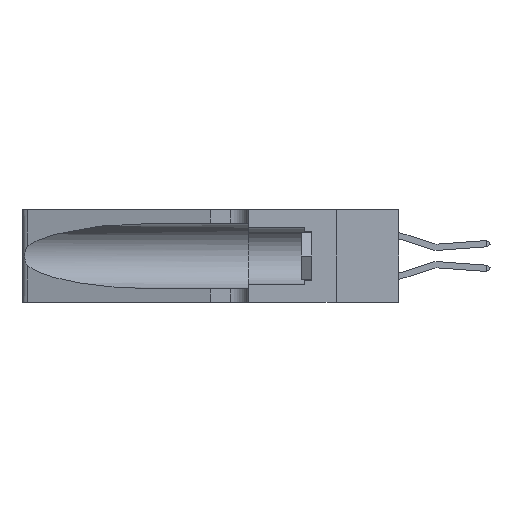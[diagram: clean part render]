
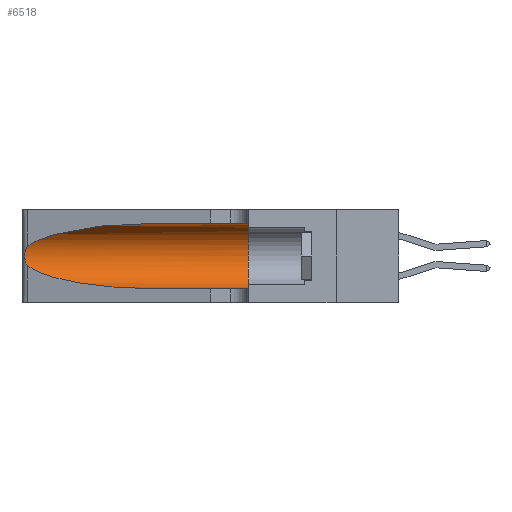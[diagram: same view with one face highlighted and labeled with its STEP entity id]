
A CAD part, left-side view. The second image highlights one B-rep face of the part: STEP entity #6518.
In plain terms, the highlighted cylindrical face has radius 3.308 mm (diameter 6.617 mm), a partial arc.
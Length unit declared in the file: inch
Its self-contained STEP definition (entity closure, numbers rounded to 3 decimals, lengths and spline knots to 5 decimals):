
#9 = B_SPLINE_CURVE_WITH_KNOTS ( 'NONE', 3,
 ( #10146, #8368, #3070, #15418, #4874, #17189, #6656, #18948, #8446, #20697, #10224, #22451, #12012, #1357 ),
 .UNSPECIFIED., .F., .F.,
 ( 4, 2, 2, 2, 2, 2, 4 ),
 ( 0., 0.00027, 0.00053, 0.00107, 0.0016, 0.00187, 0.00214 ),
 .UNSPECIFIED. ) ;
#262 = DIRECTION ( 'NONE',  ( 0., 1., 0. ) ) ;
#530 = AXIS2_PLACEMENT_3D ( 'NONE', #13227, #7877, #11489 ) ;
#1022 =( BOUNDED_CURVE ( )  B_SPLINE_CURVE ( 3, ( #15850, #14118, #1743, #5320 ),
 .UNSPECIFIED., .F., .F. ) 
 B_SPLINE_CURVE_WITH_KNOTS ( ( 4, 4 ),
 ( 1.5708, 2.84003 ),
 .UNSPECIFIED. ) 
 CURVE ( )  GEOMETRIC_REPRESENTATION_ITEM ( )  RATIONAL_B_SPLINE_CURVE ( ( 1., 0.87, 0.87, 1. ) ) 
 REPRESENTATION_ITEM ( '' )  );
#1357 = CARTESIAN_POINT ( 'NONE',  ( 0.25487, 1.22718, 0.14631 ) ) ;
#1743 = CARTESIAN_POINT ( 'NONE',  ( 0.2373, 1.15595, 0.28018 ) ) ;
#2029 = EDGE_CURVE ( 'NONE', #11776, #16020, #1022, .T. ) ;
#2551 = AXIS2_PLACEMENT_3D ( 'NONE', #10957, #262, #12705 ) ;
#2597 = ORIENTED_EDGE ( 'NONE', *, *, #8225, .T. ) ;
#2826 = FACE_OUTER_BOUND ( 'NONE', #10671, .T. ) ;
#3070 = CARTESIAN_POINT ( 'NONE',  ( 0.25639, 1.23184, 0.21858 ) ) ;
#4047 = CARTESIAN_POINT ( 'NONE',  ( 0.1305, 0.72297, 0.05475 ) ) ;
#4874 = CARTESIAN_POINT ( 'NONE',  ( 0.25854, 1.2359, 0.20912 ) ) ;
#5320 = CARTESIAN_POINT ( 'NONE',  ( 0.25487, 1.22718, 0.22369 ) ) ;
#5664 = ORIENTED_EDGE ( 'NONE', *, *, #8395, .F. ) ;
#6165 = DIRECTION ( 'NONE',  ( 0., -1., 0. ) ) ;
#6518 = ADVANCED_FACE ( 'NONE', ( #2826 ), #11759, .F. ) ;
#6656 = CARTESIAN_POINT ( 'NONE',  ( 0.26075, 1.23896, 0.19203 ) ) ;
#7087 = CARTESIAN_POINT ( 'NONE',  ( 0.25487, 1.22718, 0.22369 ) ) ;
#7181 = ORIENTED_EDGE ( 'NONE', *, *, #8747, .F. ) ;
#7194 = CARTESIAN_POINT ( 'NONE',  ( 0.18966, 0.96281, 0.05475 ) ) ;
#7877 = DIRECTION ( 'NONE',  ( 0., -1., 0. ) ) ;
#8013 = CIRCLE ( 'NONE', #2551, 0.13025 ) ;
#8225 = EDGE_CURVE ( 'NONE', #18808, #12604, #9171, .T. ) ;
#8368 = CARTESIAN_POINT ( 'NONE',  ( 0.25555, 1.22994, 0.2215 ) ) ;
#8395 = EDGE_CURVE ( 'NONE', #11776, #13294, #14104, .T. ) ;
#8446 = CARTESIAN_POINT ( 'NONE',  ( 0.26017, 1.23833, 0.17102 ) ) ;
#8747 = EDGE_CURVE ( 'NONE', #13294, #12604, #8013, .T. ) ;
#8905 = CARTESIAN_POINT ( 'NONE',  ( 0.1305, 0.72297, 0.31525 ) ) ;
#9171 = LINE ( 'NONE', #18378, #17946 ) ;
#9977 = VECTOR ( 'NONE', #11907, 39.37008 ) ;
#10146 = CARTESIAN_POINT ( 'NONE',  ( 0.25487, 1.22718, 0.22369 ) ) ;
#10177 =( BOUNDED_CURVE ( )  B_SPLINE_CURVE ( 3, ( #15953, #17741, #7194, #19487 ),
 .UNSPECIFIED., .F., .F. ) 
 B_SPLINE_CURVE_WITH_KNOTS ( ( 4, 4 ),
 ( 3.44316, 4.71239 ),
 .UNSPECIFIED. ) 
 CURVE ( )  GEOMETRIC_REPRESENTATION_ITEM ( )  RATIONAL_B_SPLINE_CURVE ( ( 1., 0.87, 0.87, 1. ) ) 
 REPRESENTATION_ITEM ( '' )  );
#10224 = CARTESIAN_POINT ( 'NONE',  ( 0.25789, 1.23486, 0.15765 ) ) ;
#10671 = EDGE_LOOP ( 'NONE', ( #17252, #17301, #17947, #2597, #7181, #5664 ) ) ;
#10957 = CARTESIAN_POINT ( 'NONE',  ( 0.1305, 0.35, 0.185 ) ) ;
#11489 = DIRECTION ( 'NONE',  ( 0., 0., -1. ) ) ;
#11645 = EDGE_CURVE ( 'NONE', #16020, #13920, #9, .T. ) ;
#11759 = CYLINDRICAL_SURFACE ( 'NONE', #530, 0.13025 ) ;
#11776 = VERTEX_POINT ( 'NONE', #8905 ) ;
#11907 = DIRECTION ( 'NONE',  ( 0., -1., 0. ) ) ;
#12012 = CARTESIAN_POINT ( 'NONE',  ( 0.25555, 1.22993, 0.14849 ) ) ;
#12604 = VERTEX_POINT ( 'NONE', #21870 ) ;
#12705 = DIRECTION ( 'NONE',  ( 0., 0., 1. ) ) ;
#13227 = CARTESIAN_POINT ( 'NONE',  ( 0.1305, 1.61858, 0.185 ) ) ;
#13294 = VERTEX_POINT ( 'NONE', #18485 ) ;
#13920 = VERTEX_POINT ( 'NONE', #14878 ) ;
#14104 = LINE ( 'NONE', #22343, #9977 ) ;
#14118 = CARTESIAN_POINT ( 'NONE',  ( 0.18966, 0.96281, 0.31525 ) ) ;
#14878 = CARTESIAN_POINT ( 'NONE',  ( 0.25487, 1.22718, 0.14631 ) ) ;
#15418 = CARTESIAN_POINT ( 'NONE',  ( 0.25787, 1.23484, 0.2124 ) ) ;
#15850 = CARTESIAN_POINT ( 'NONE',  ( 0.1305, 0.72297, 0.31525 ) ) ;
#15953 = CARTESIAN_POINT ( 'NONE',  ( 0.25487, 1.22718, 0.14631 ) ) ;
#16020 = VERTEX_POINT ( 'NONE', #7087 ) ;
#17189 = CARTESIAN_POINT ( 'NONE',  ( 0.26018, 1.23835, 0.19895 ) ) ;
#17252 = ORIENTED_EDGE ( 'NONE', *, *, #2029, .T. ) ;
#17301 = ORIENTED_EDGE ( 'NONE', *, *, #11645, .T. ) ;
#17321 = EDGE_CURVE ( 'NONE', #13920, #18808, #10177, .T. ) ;
#17741 = CARTESIAN_POINT ( 'NONE',  ( 0.2373, 1.15595, 0.08982 ) ) ;
#17946 = VECTOR ( 'NONE', #6165, 39.37008 ) ;
#17947 = ORIENTED_EDGE ( 'NONE', *, *, #17321, .T. ) ;
#18378 = CARTESIAN_POINT ( 'NONE',  ( 0.1305, 1.61858, 0.05475 ) ) ;
#18485 = CARTESIAN_POINT ( 'NONE',  ( 0.1305, 0.35, 0.31525 ) ) ;
#18808 = VERTEX_POINT ( 'NONE', #4047 ) ;
#18948 = CARTESIAN_POINT ( 'NONE',  ( 0.26075, 1.23896, 0.178 ) ) ;
#19487 = CARTESIAN_POINT ( 'NONE',  ( 0.1305, 0.72297, 0.05475 ) ) ;
#20697 = CARTESIAN_POINT ( 'NONE',  ( 0.25856, 1.23593, 0.16098 ) ) ;
#21870 = CARTESIAN_POINT ( 'NONE',  ( 0.1305, 0.35, 0.05475 ) ) ;
#22343 = CARTESIAN_POINT ( 'NONE',  ( 0.1305, 1.61858, 0.31525 ) ) ;
#22451 = CARTESIAN_POINT ( 'NONE',  ( 0.25639, 1.23186, 0.15144 ) ) ;
